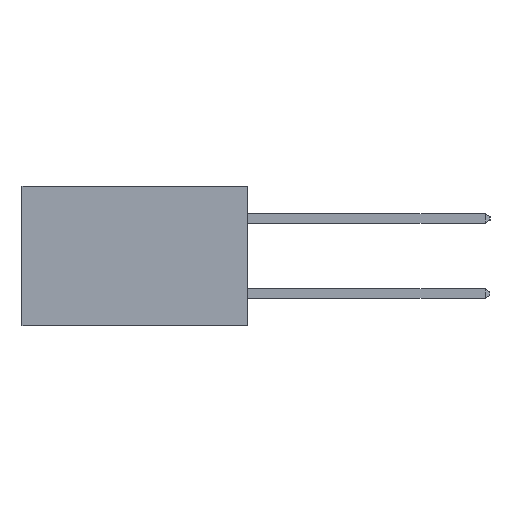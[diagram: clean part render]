
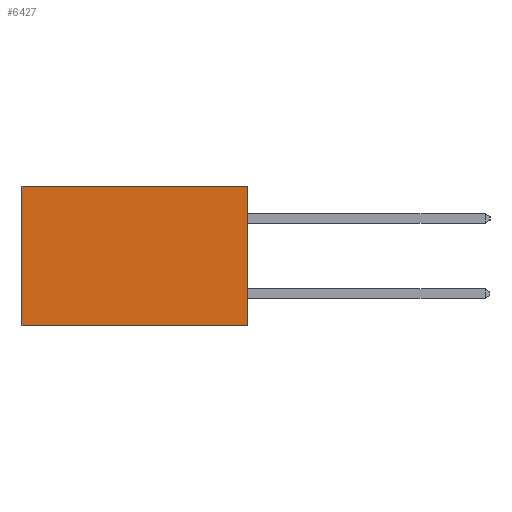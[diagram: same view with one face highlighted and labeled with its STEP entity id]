
A CAD part, left-side view. The second image highlights one B-rep face of the part: STEP entity #6427.
In plain terms, the highlighted planar face has unit normal (-1, 0, 0).
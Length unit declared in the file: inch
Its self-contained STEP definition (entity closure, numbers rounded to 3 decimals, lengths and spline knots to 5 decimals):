
#473 = ORIENTED_EDGE ( 'NONE', *, *, #15524, .F. ) ;
#757 = DIRECTION ( 'NONE',  ( 0., 0., -1. ) ) ;
#1163 = LINE ( 'NONE', #17855, #4181 ) ;
#1473 = VERTEX_POINT ( 'NONE', #16031 ) ;
#3455 = CARTESIAN_POINT ( 'NONE',  ( 0.298, 0.6, 0. ) ) ;
#3494 = EDGE_CURVE ( 'NONE', #15568, #8667, #9076, .T. ) ;
#4143 = CARTESIAN_POINT ( 'NONE',  ( 0.298, 0., 0. ) ) ;
#4181 = VECTOR ( 'NONE', #6173, 39.37008 ) ;
#4533 = DIRECTION ( 'NONE',  ( 1., 0., 0. ) ) ;
#4681 = DIRECTION ( 'NONE',  ( 0., 0., -1. ) ) ;
#5105 = LINE ( 'NONE', #7286, #12366 ) ;
#5543 = CARTESIAN_POINT ( 'NONE',  ( 0.298, 0.6, -0.37 ) ) ;
#5950 = VERTEX_POINT ( 'NONE', #3455 ) ;
#6017 = EDGE_CURVE ( 'NONE', #5950, #8667, #17754, .T. ) ;
#6173 = DIRECTION ( 'NONE',  ( 0., 1., 0. ) ) ;
#6427 = ADVANCED_FACE ( 'NONE', ( #18609 ), #15256, .F. ) ;
#7286 = CARTESIAN_POINT ( 'NONE',  ( 0.298, 0., 0. ) ) ;
#7843 = CARTESIAN_POINT ( 'NONE',  ( 0.298, 0.6, 0. ) ) ;
#8667 = VERTEX_POINT ( 'NONE', #5543 ) ;
#8739 = DIRECTION ( 'NONE',  ( 0., 0., -1. ) ) ;
#9076 = LINE ( 'NONE', #16662, #9530 ) ;
#9530 = VECTOR ( 'NONE', #15697, 39.37008 ) ;
#9790 = ORIENTED_EDGE ( 'NONE', *, *, #12497, .T. ) ;
#10279 = CARTESIAN_POINT ( 'NONE',  ( 0.298, 0., -0.37 ) ) ;
#10313 = ORIENTED_EDGE ( 'NONE', *, *, #3494, .F. ) ;
#11615 = AXIS2_PLACEMENT_3D ( 'NONE', #4143, #4533, #4681 ) ;
#12366 = VECTOR ( 'NONE', #8739, 39.37008 ) ;
#12497 = EDGE_CURVE ( 'NONE', #1473, #5950, #1163, .T. ) ;
#13542 = VECTOR ( 'NONE', #757, 39.37008 ) ;
#15256 = PLANE ( 'NONE',  #11615 ) ;
#15524 = EDGE_CURVE ( 'NONE', #1473, #15568, #5105, .T. ) ;
#15568 = VERTEX_POINT ( 'NONE', #10279 ) ;
#15697 = DIRECTION ( 'NONE',  ( 0., 1., 0. ) ) ;
#16031 = CARTESIAN_POINT ( 'NONE',  ( 0.298, 0., 0. ) ) ;
#16384 = ORIENTED_EDGE ( 'NONE', *, *, #6017, .T. ) ;
#16662 = CARTESIAN_POINT ( 'NONE',  ( 0.298, 0., -0.37 ) ) ;
#17754 = LINE ( 'NONE', #7843, #13542 ) ;
#17855 = CARTESIAN_POINT ( 'NONE',  ( 0.298, 0., 0. ) ) ;
#18506 = EDGE_LOOP ( 'NONE', ( #16384, #10313, #473, #9790 ) ) ;
#18609 = FACE_OUTER_BOUND ( 'NONE', #18506, .T. ) ;
